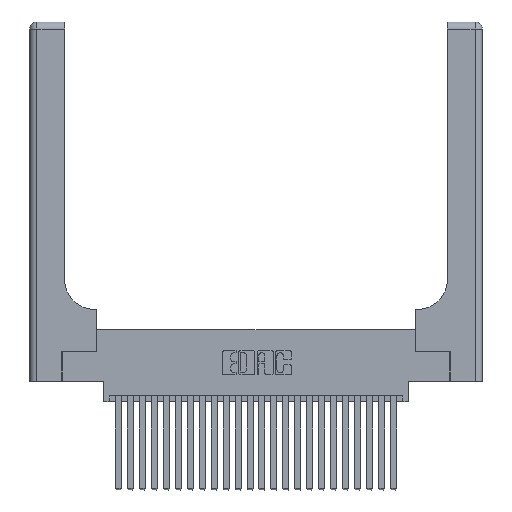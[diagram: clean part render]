
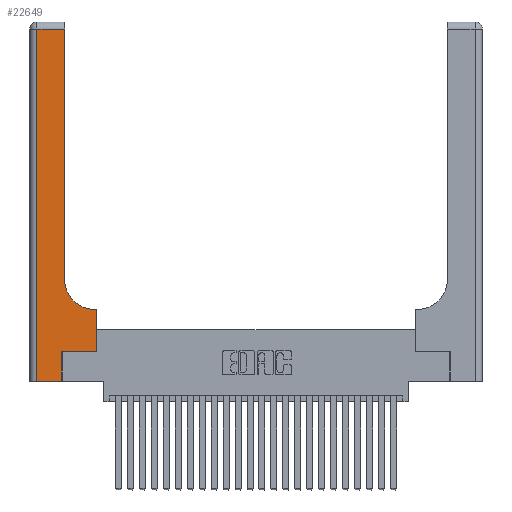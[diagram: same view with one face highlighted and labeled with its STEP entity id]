
A CAD part, top view. The second image highlights one B-rep face of the part: STEP entity #22649.
In plain terms, the highlighted planar face has unit normal (0, 0, 1).
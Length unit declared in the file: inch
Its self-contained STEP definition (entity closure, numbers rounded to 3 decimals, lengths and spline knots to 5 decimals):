
#333 = LINE ( 'NONE', #10135, #10240 ) ;
#621 = VERTEX_POINT ( 'NONE', #3927 ) ;
#807 = DIRECTION ( 'NONE',  ( 1., 0., 0. ) ) ;
#1313 = VECTOR ( 'NONE', #20494, 39.37008 ) ;
#1399 = EDGE_CURVE ( 'NONE', #6861, #10077, #23361, .T. ) ;
#2005 = DIRECTION ( 'NONE',  ( -1., 0., 0. ) ) ;
#2453 = PLANE ( 'NONE',  #8992 ) ;
#2763 = CARTESIAN_POINT ( 'NONE',  ( 0.06, 2.94, 0.37 ) ) ;
#3927 = CARTESIAN_POINT ( 'NONE',  ( 0.2915, 0.85, 0.37 ) ) ;
#4911 = VECTOR ( 'NONE', #15231, 39.37008 ) ;
#5246 = LINE ( 'NONE', #16237, #21433 ) ;
#6095 = CARTESIAN_POINT ( 'NONE',  ( 0.269, 0.25, 0.37 ) ) ;
#6297 = CARTESIAN_POINT ( 'NONE',  ( 0.269, 0., 0.37 ) ) ;
#6710 = DIRECTION ( 'NONE',  ( -1., 0., 0. ) ) ;
#6861 = VERTEX_POINT ( 'NONE', #25516 ) ;
#6924 = EDGE_CURVE ( 'NONE', #16116, #11724, #7663, .T. ) ;
#7013 = ORIENTED_EDGE ( 'NONE', *, *, #1399, .T. ) ;
#7663 = LINE ( 'NONE', #13919, #17274 ) ;
#7904 = EDGE_CURVE ( 'NONE', #11724, #23918, #333, .T. ) ;
#8571 = EDGE_CURVE ( 'NONE', #23918, #21436, #23050, .T. ) ;
#8817 = LINE ( 'NONE', #26295, #18962 ) ;
#8931 = ORIENTED_EDGE ( 'NONE', *, *, #25987, .T. ) ;
#8992 = AXIS2_PLACEMENT_3D ( 'NONE', #24737, #18894, #6710 ) ;
#9075 = VERTEX_POINT ( 'NONE', #25875 ) ;
#10077 = VERTEX_POINT ( 'NONE', #15388 ) ;
#10135 = CARTESIAN_POINT ( 'NONE',  ( 0., 0., 0.37 ) ) ;
#10170 = ORIENTED_EDGE ( 'NONE', *, *, #22906, .T. ) ;
#10240 = VECTOR ( 'NONE', #18611, 39.37008 ) ;
#10713 = ORIENTED_EDGE ( 'NONE', *, *, #25140, .T. ) ;
#11094 = CARTESIAN_POINT ( 'NONE',  ( 0.269, 0., 0.37 ) ) ;
#11247 = EDGE_CURVE ( 'NONE', #10077, #22001, #15825, .T. ) ;
#11724 = VERTEX_POINT ( 'NONE', #16623 ) ;
#13352 = DIRECTION ( 'NONE',  ( 0., 0., -1. ) ) ;
#13919 = CARTESIAN_POINT ( 'NONE',  ( 0.06, 3., 0.37 ) ) ;
#14057 = VECTOR ( 'NONE', #15762, 39.37008 ) ;
#14844 = CARTESIAN_POINT ( 'NONE',  ( 0.5415, 0.6, 0.37 ) ) ;
#15231 = DIRECTION ( 'NONE',  ( -1., 0., 0. ) ) ;
#15388 = CARTESIAN_POINT ( 'NONE',  ( 0.5585, 0.6, 0.37 ) ) ;
#15762 = DIRECTION ( 'NONE',  ( 0., 1., 0. ) ) ;
#15787 = CARTESIAN_POINT ( 'NONE',  ( 0.5585, 0.25, 0.37 ) ) ;
#15825 = LINE ( 'NONE', #17255, #4911 ) ;
#15930 = DIRECTION ( 'NONE',  ( 0., -1., 0. ) ) ;
#16012 = CARTESIAN_POINT ( 'NONE',  ( 0.2915, 3., 0.37 ) ) ;
#16116 = VERTEX_POINT ( 'NONE', #2763 ) ;
#16237 = CARTESIAN_POINT ( 'NONE',  ( 0.269, 0.25, 0.37 ) ) ;
#16623 = CARTESIAN_POINT ( 'NONE',  ( 0.06, 0., 0.37 ) ) ;
#16629 = VECTOR ( 'NONE', #19571, 39.37008 ) ;
#17255 = CARTESIAN_POINT ( 'NONE',  ( 0.2915, 0.6, 0.37 ) ) ;
#17274 = VECTOR ( 'NONE', #15930, 39.37008 ) ;
#17568 = FACE_OUTER_BOUND ( 'NONE', #19784, .T. ) ;
#17857 = LINE ( 'NONE', #16012, #16629 ) ;
#18228 = DIRECTION ( 'NONE',  ( 1., 0., 0. ) ) ;
#18611 = DIRECTION ( 'NONE',  ( 1., 0., 0. ) ) ;
#18894 = DIRECTION ( 'NONE',  ( 0., 0., -1. ) ) ;
#18962 = VECTOR ( 'NONE', #2005, 39.37008 ) ;
#19427 = ORIENTED_EDGE ( 'NONE', *, *, #26068, .T. ) ;
#19571 = DIRECTION ( 'NONE',  ( 0., 1., 0. ) ) ;
#19784 = EDGE_LOOP ( 'NONE', ( #10170, #19427, #26335, #21568, #22369, #8931, #7013, #22806, #10713 ) ) ;
#20494 = DIRECTION ( 'NONE',  ( 0., 1., 0. ) ) ;
#21433 = VECTOR ( 'NONE', #18228, 39.37008 ) ;
#21436 = VERTEX_POINT ( 'NONE', #6095 ) ;
#21568 = ORIENTED_EDGE ( 'NONE', *, *, #7904, .T. ) ;
#22001 = VERTEX_POINT ( 'NONE', #14844 ) ;
#22369 = ORIENTED_EDGE ( 'NONE', *, *, #8571, .T. ) ;
#22649 = ADVANCED_FACE ( 'NONE', ( #17568 ), #2453, .F. ) ;
#22806 = ORIENTED_EDGE ( 'NONE', *, *, #11247, .T. ) ;
#22906 = EDGE_CURVE ( 'NONE', #621, #9075, #17857, .T. ) ;
#22999 = AXIS2_PLACEMENT_3D ( 'NONE', #25226, #13352, #807 ) ;
#23050 = LINE ( 'NONE', #6297, #1313 ) ;
#23361 = LINE ( 'NONE', #15787, #14057 ) ;
#23918 = VERTEX_POINT ( 'NONE', #11094 ) ;
#24737 = CARTESIAN_POINT ( 'NONE',  ( 0., 3., 0.37 ) ) ;
#24864 = CIRCLE ( 'NONE', #22999, 0.25 ) ;
#25140 = EDGE_CURVE ( 'NONE', #22001, #621, #24864, .T. ) ;
#25226 = CARTESIAN_POINT ( 'NONE',  ( 0.5415, 0.85, 0.37 ) ) ;
#25516 = CARTESIAN_POINT ( 'NONE',  ( 0.5585, 0.25, 0.37 ) ) ;
#25875 = CARTESIAN_POINT ( 'NONE',  ( 0.2915, 2.94, 0.37 ) ) ;
#25987 = EDGE_CURVE ( 'NONE', #21436, #6861, #5246, .T. ) ;
#26068 = EDGE_CURVE ( 'NONE', #9075, #16116, #8817, .T. ) ;
#26295 = CARTESIAN_POINT ( 'NONE',  ( 0., 2.94, 0.37 ) ) ;
#26335 = ORIENTED_EDGE ( 'NONE', *, *, #6924, .T. ) ;
